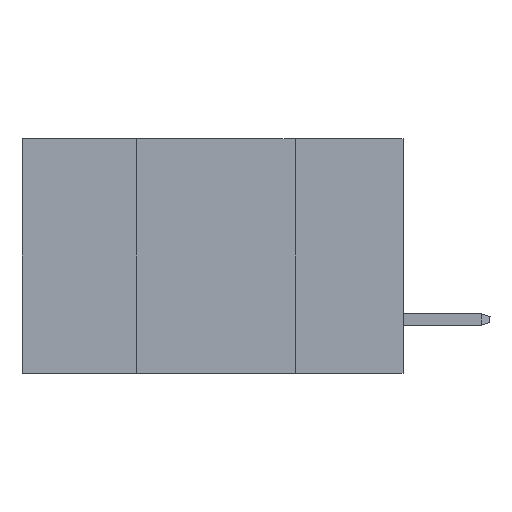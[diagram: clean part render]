
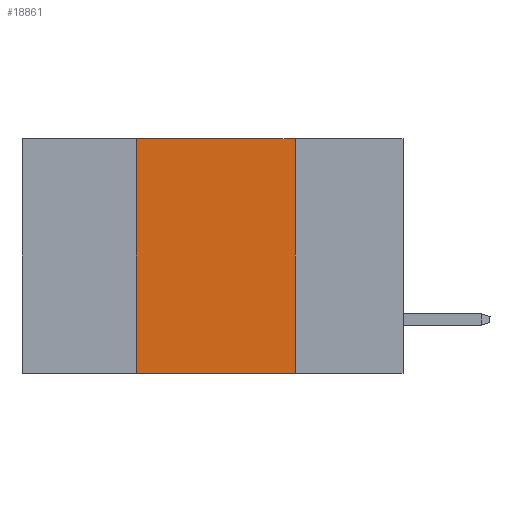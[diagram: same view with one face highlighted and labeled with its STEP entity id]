
A CAD part, left-side view. The second image highlights one B-rep face of the part: STEP entity #18861.
In plain terms, the highlighted planar face has unit normal (-1, 0, 0).
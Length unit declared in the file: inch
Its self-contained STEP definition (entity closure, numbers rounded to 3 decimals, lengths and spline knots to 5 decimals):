
#439 = LINE ( 'NONE', #4354, #11942 ) ;
#836 = VERTEX_POINT ( 'NONE', #15594 ) ;
#1167 = CARTESIAN_POINT ( 'NONE',  ( 0., 0.17, 0. ) ) ;
#1546 = VERTEX_POINT ( 'NONE', #26826 ) ;
#3652 = EDGE_CURVE ( 'NONE', #1546, #7821, #4275, .T. ) ;
#4139 = DIRECTION ( 'NONE',  ( 0., -1., 0. ) ) ;
#4215 = ORIENTED_EDGE ( 'NONE', *, *, #18909, .T. ) ;
#4275 = LINE ( 'NONE', #26176, #9279 ) ;
#4354 = CARTESIAN_POINT ( 'NONE',  ( 0., 0.42, 0. ) ) ;
#5620 = CARTESIAN_POINT ( 'NONE',  ( 0., 0.17, 0. ) ) ;
#5644 = ORIENTED_EDGE ( 'NONE', *, *, #3652, .F. ) ;
#6185 = DIRECTION ( 'NONE',  ( 1., 0., 0. ) ) ;
#6481 = DIRECTION ( 'NONE',  ( 0., 0., -1. ) ) ;
#7821 = VERTEX_POINT ( 'NONE', #5620 ) ;
#7987 = LINE ( 'NONE', #1167, #16753 ) ;
#8015 = DIRECTION ( 'NONE',  ( 0., -1., 0. ) ) ;
#9279 = VECTOR ( 'NONE', #4139, 39.37008 ) ;
#9299 = DIRECTION ( 'NONE',  ( 0., 0., 1. ) ) ;
#11942 = VECTOR ( 'NONE', #9299, 39.37008 ) ;
#12734 = PLANE ( 'NONE',  #18323 ) ;
#12888 = FACE_OUTER_BOUND ( 'NONE', #16740, .T. ) ;
#13067 = EDGE_CURVE ( 'NONE', #7821, #836, #7987, .T. ) ;
#13981 = ORIENTED_EDGE ( 'NONE', *, *, #28269, .F. ) ;
#15594 = CARTESIAN_POINT ( 'NONE',  ( 0., 0.17, -0.37 ) ) ;
#16740 = EDGE_LOOP ( 'NONE', ( #25562, #5644, #13981, #4215 ) ) ;
#16753 = VECTOR ( 'NONE', #25680, 39.37008 ) ;
#18266 = VERTEX_POINT ( 'NONE', #25555 ) ;
#18323 = AXIS2_PLACEMENT_3D ( 'NONE', #21566, #6185, #6481 ) ;
#18861 = ADVANCED_FACE ( 'NONE', ( #12888 ), #12734, .F. ) ;
#18909 = EDGE_CURVE ( 'NONE', #18266, #836, #19841, .T. ) ;
#19841 = LINE ( 'NONE', #28681, #22491 ) ;
#21566 = CARTESIAN_POINT ( 'NONE',  ( 0., 0.6, 0. ) ) ;
#22491 = VECTOR ( 'NONE', #8015, 39.37008 ) ;
#25555 = CARTESIAN_POINT ( 'NONE',  ( 0., 0.42, -0.37 ) ) ;
#25562 = ORIENTED_EDGE ( 'NONE', *, *, #13067, .F. ) ;
#25680 = DIRECTION ( 'NONE',  ( 0., 0., -1. ) ) ;
#26176 = CARTESIAN_POINT ( 'NONE',  ( 0., 0.6, 0. ) ) ;
#26826 = CARTESIAN_POINT ( 'NONE',  ( 0., 0.42, 0. ) ) ;
#28269 = EDGE_CURVE ( 'NONE', #18266, #1546, #439, .T. ) ;
#28681 = CARTESIAN_POINT ( 'NONE',  ( 0., 0.6, -0.37 ) ) ;
